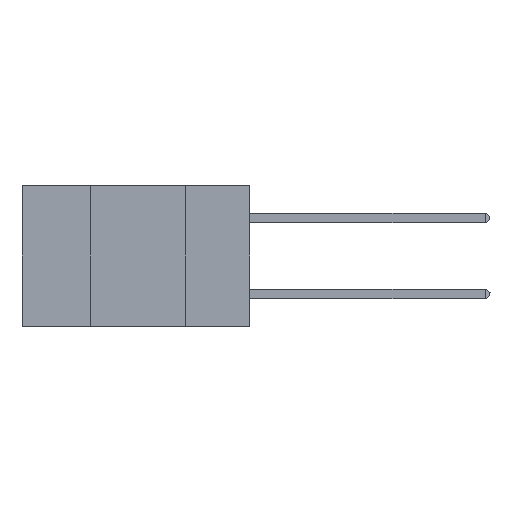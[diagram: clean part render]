
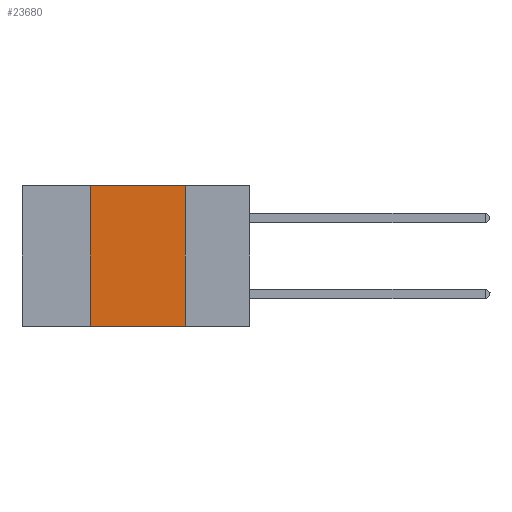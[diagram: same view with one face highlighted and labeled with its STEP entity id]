
A CAD part, left-side view. The second image highlights one B-rep face of the part: STEP entity #23680.
In plain terms, the highlighted planar face has unit normal (-1, 0, 0).
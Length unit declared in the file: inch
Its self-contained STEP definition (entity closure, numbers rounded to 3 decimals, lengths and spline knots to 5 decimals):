
#77 = DIRECTION ( 'NONE',  ( 0., 0., -1. ) ) ;
#88 = FACE_OUTER_BOUND ( 'NONE', #14588, .T. ) ;
#327 = ORIENTED_EDGE ( 'NONE', *, *, #22903, .F. ) ;
#604 = CARTESIAN_POINT ( 'NONE',  ( 0., 0.17, 0. ) ) ;
#1203 = DIRECTION ( 'NONE',  ( 0., 0., -1. ) ) ;
#1251 = CARTESIAN_POINT ( 'NONE',  ( 0., 0.17, -0.37 ) ) ;
#2141 = CARTESIAN_POINT ( 'NONE',  ( 0., 0.6, 0. ) ) ;
#2217 = EDGE_CURVE ( 'NONE', #24953, #21559, #17349, .T. ) ;
#2299 = VECTOR ( 'NONE', #13618, 39.37008 ) ;
#3773 = CARTESIAN_POINT ( 'NONE',  ( 0., 0.17, 0. ) ) ;
#5059 = LINE ( 'NONE', #13870, #2299 ) ;
#6118 = EDGE_CURVE ( 'NONE', #24953, #17396, #21592, .T. ) ;
#6791 = DIRECTION ( 'NONE',  ( 0., 0., 1. ) ) ;
#9605 = ORIENTED_EDGE ( 'NONE', *, *, #2217, .T. ) ;
#10223 = ORIENTED_EDGE ( 'NONE', *, *, #11549, .F. ) ;
#11549 = EDGE_CURVE ( 'NONE', #17396, #22690, #5059, .T. ) ;
#13618 = DIRECTION ( 'NONE',  ( 0., -1., 0. ) ) ;
#13870 = CARTESIAN_POINT ( 'NONE',  ( 0., 0.6, 0. ) ) ;
#14269 = AXIS2_PLACEMENT_3D ( 'NONE', #2141, #21446, #77 ) ;
#14588 = EDGE_LOOP ( 'NONE', ( #327, #10223, #22099, #9605 ) ) ;
#15499 = PLANE ( 'NONE',  #14269 ) ;
#15933 = CARTESIAN_POINT ( 'NONE',  ( 0., 0.42, 0. ) ) ;
#16318 = VECTOR ( 'NONE', #1203, 39.37008 ) ;
#17349 = LINE ( 'NONE', #20647, #21014 ) ;
#17396 = VERTEX_POINT ( 'NONE', #15933 ) ;
#20230 = CARTESIAN_POINT ( 'NONE',  ( 0., 0.42, 0. ) ) ;
#20647 = CARTESIAN_POINT ( 'NONE',  ( 0., 0.6, -0.37 ) ) ;
#21014 = VECTOR ( 'NONE', #22417, 39.37008 ) ;
#21446 = DIRECTION ( 'NONE',  ( 1., 0., 0. ) ) ;
#21559 = VERTEX_POINT ( 'NONE', #1251 ) ;
#21592 = LINE ( 'NONE', #20230, #22502 ) ;
#22099 = ORIENTED_EDGE ( 'NONE', *, *, #6118, .F. ) ;
#22417 = DIRECTION ( 'NONE',  ( 0., -1., 0. ) ) ;
#22502 = VECTOR ( 'NONE', #6791, 39.37008 ) ;
#22690 = VERTEX_POINT ( 'NONE', #3773 ) ;
#22725 = CARTESIAN_POINT ( 'NONE',  ( 0., 0.42, -0.37 ) ) ;
#22903 = EDGE_CURVE ( 'NONE', #22690, #21559, #23637, .T. ) ;
#23637 = LINE ( 'NONE', #604, #16318 ) ;
#23680 = ADVANCED_FACE ( 'NONE', ( #88 ), #15499, .F. ) ;
#24953 = VERTEX_POINT ( 'NONE', #22725 ) ;
